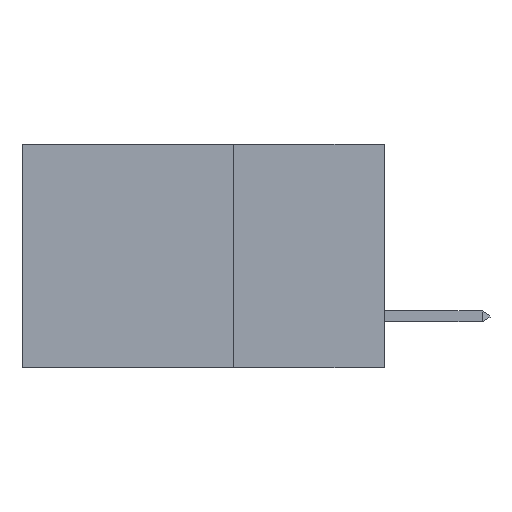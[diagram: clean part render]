
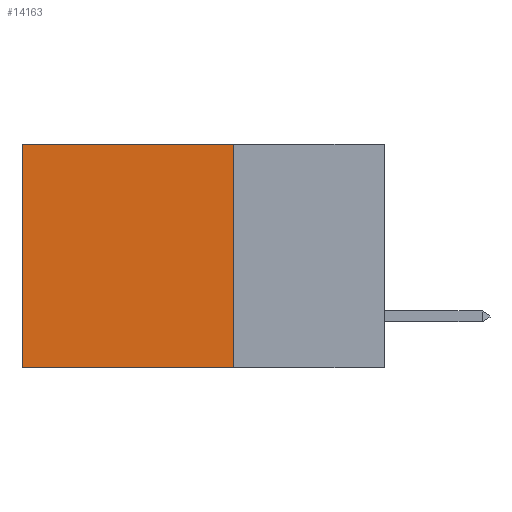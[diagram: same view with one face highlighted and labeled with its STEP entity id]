
A CAD part, left-side view. The second image highlights one B-rep face of the part: STEP entity #14163.
In plain terms, the highlighted planar face has unit normal (-1, 0, 0).
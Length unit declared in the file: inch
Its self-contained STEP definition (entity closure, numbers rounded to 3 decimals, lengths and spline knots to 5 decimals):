
#756 = ORIENTED_EDGE ( 'NONE', *, *, #10026, .T. ) ;
#1023 = LINE ( 'NONE', #12724, #4735 ) ;
#1159 = DIRECTION ( 'NONE',  ( 0., 0., -1. ) ) ;
#1362 = DIRECTION ( 'NONE',  ( 0., 1., 0. ) ) ;
#1599 = CARTESIAN_POINT ( 'NONE',  ( 0.2875, 0.6, 0. ) ) ;
#1757 = LINE ( 'NONE', #1599, #14512 ) ;
#1838 = PLANE ( 'NONE',  #9917 ) ;
#2199 = EDGE_CURVE ( 'NONE', #11297, #2507, #10213, .T. ) ;
#2507 = VERTEX_POINT ( 'NONE', #9610 ) ;
#3062 = ORIENTED_EDGE ( 'NONE', *, *, #13924, .F. ) ;
#3116 = VECTOR ( 'NONE', #16120, 39.37008 ) ;
#3216 = DIRECTION ( 'NONE',  ( 1., 0., 0. ) ) ;
#3535 = CARTESIAN_POINT ( 'NONE',  ( 0.2875, 0.6, -0.37 ) ) ;
#4735 = VECTOR ( 'NONE', #1362, 39.37008 ) ;
#4918 = ORIENTED_EDGE ( 'NONE', *, *, #2199, .T. ) ;
#5701 = EDGE_CURVE ( 'NONE', #11297, #5798, #11201, .T. ) ;
#5798 = VERTEX_POINT ( 'NONE', #14194 ) ;
#6709 = ORIENTED_EDGE ( 'NONE', *, *, #5701, .F. ) ;
#7871 = CARTESIAN_POINT ( 'NONE',  ( 0.2875, 0.25, 0. ) ) ;
#8458 = FACE_OUTER_BOUND ( 'NONE', #8723, .T. ) ;
#8723 = EDGE_LOOP ( 'NONE', ( #756, #3062, #6709, #4918 ) ) ;
#9252 = CARTESIAN_POINT ( 'NONE',  ( 0.2875, 0.25, 0. ) ) ;
#9610 = CARTESIAN_POINT ( 'NONE',  ( 0.2875, 0.6, 0. ) ) ;
#9666 = DIRECTION ( 'NONE',  ( 0., 0., -1. ) ) ;
#9917 = AXIS2_PLACEMENT_3D ( 'NONE', #11098, #3216, #12324 ) ;
#10026 = EDGE_CURVE ( 'NONE', #2507, #15676, #1757, .T. ) ;
#10213 = LINE ( 'NONE', #14496, #3116 ) ;
#11098 = CARTESIAN_POINT ( 'NONE',  ( 0.2875, 0.25, 0. ) ) ;
#11201 = LINE ( 'NONE', #9252, #14278 ) ;
#11297 = VERTEX_POINT ( 'NONE', #7871 ) ;
#12324 = DIRECTION ( 'NONE',  ( 0., 0., -1. ) ) ;
#12724 = CARTESIAN_POINT ( 'NONE',  ( 0.2875, 0.25, -0.37 ) ) ;
#13924 = EDGE_CURVE ( 'NONE', #5798, #15676, #1023, .T. ) ;
#14163 = ADVANCED_FACE ( 'NONE', ( #8458 ), #1838, .F. ) ;
#14194 = CARTESIAN_POINT ( 'NONE',  ( 0.2875, 0.25, -0.37 ) ) ;
#14278 = VECTOR ( 'NONE', #1159, 39.37008 ) ;
#14496 = CARTESIAN_POINT ( 'NONE',  ( 0.2875, 0.25, 0. ) ) ;
#14512 = VECTOR ( 'NONE', #9666, 39.37008 ) ;
#15676 = VERTEX_POINT ( 'NONE', #3535 ) ;
#16120 = DIRECTION ( 'NONE',  ( 0., 1., 0. ) ) ;
